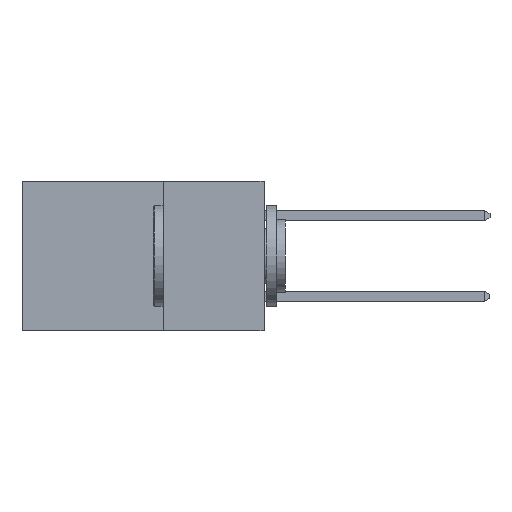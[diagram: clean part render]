
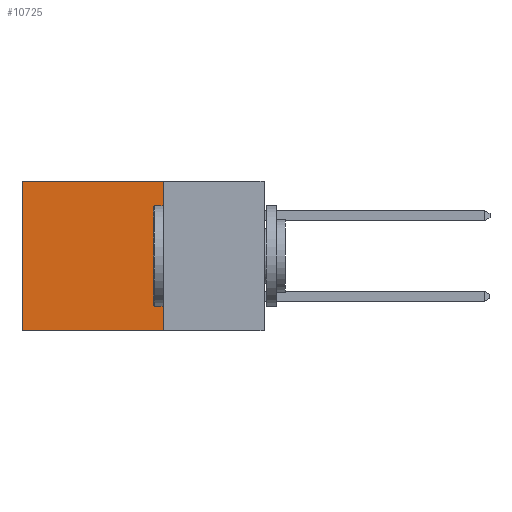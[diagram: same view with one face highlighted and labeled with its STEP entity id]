
A CAD part, left-side view. The second image highlights one B-rep face of the part: STEP entity #10725.
In plain terms, the highlighted planar face has unit normal (-1, 0, 0).
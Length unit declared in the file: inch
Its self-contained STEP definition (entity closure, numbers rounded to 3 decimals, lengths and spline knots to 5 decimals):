
#229 = DIRECTION ( 'NONE',  ( 0., 0., -1. ) ) ;
#1566 = CARTESIAN_POINT ( 'NONE',  ( 0.298, 0.25, 0. ) ) ;
#3342 = VECTOR ( 'NONE', #15782, 39.37008 ) ;
#3769 = LINE ( 'NONE', #6173, #3342 ) ;
#4072 = DIRECTION ( 'NONE',  ( 0., 1., 0. ) ) ;
#4137 = EDGE_CURVE ( 'NONE', #8385, #11185, #16039, .T. ) ;
#5126 = CARTESIAN_POINT ( 'NONE',  ( 0.298, 0.25, 0. ) ) ;
#6173 = CARTESIAN_POINT ( 'NONE',  ( 0.298, 0.6, 0. ) ) ;
#6237 = FACE_OUTER_BOUND ( 'NONE', #8114, .T. ) ;
#6563 = DIRECTION ( 'NONE',  ( 0., 0., -1. ) ) ;
#7014 = CARTESIAN_POINT ( 'NONE',  ( 0.298, 0.6, -0.37 ) ) ;
#7054 = LINE ( 'NONE', #11032, #10706 ) ;
#7848 = ORIENTED_EDGE ( 'NONE', *, *, #14014, .T. ) ;
#8114 = EDGE_LOOP ( 'NONE', ( #7848, #8485, #8613, #9883 ) ) ;
#8181 = CARTESIAN_POINT ( 'NONE',  ( 0.298, 0.25, -0.37 ) ) ;
#8225 = VECTOR ( 'NONE', #13657, 39.37008 ) ;
#8385 = VERTEX_POINT ( 'NONE', #1566 ) ;
#8485 = ORIENTED_EDGE ( 'NONE', *, *, #12906, .F. ) ;
#8613 = ORIENTED_EDGE ( 'NONE', *, *, #4137, .F. ) ;
#8800 = VECTOR ( 'NONE', #229, 39.37008 ) ;
#9276 = PLANE ( 'NONE',  #17510 ) ;
#9883 = ORIENTED_EDGE ( 'NONE', *, *, #11575, .T. ) ;
#10127 = CARTESIAN_POINT ( 'NONE',  ( 0.298, 0.25, -0.37 ) ) ;
#10706 = VECTOR ( 'NONE', #4072, 39.37008 ) ;
#10725 = ADVANCED_FACE ( 'NONE', ( #6237 ), #9276, .F. ) ;
#10964 = VERTEX_POINT ( 'NONE', #7014 ) ;
#11032 = CARTESIAN_POINT ( 'NONE',  ( 0.298, 0.25, 0. ) ) ;
#11185 = VERTEX_POINT ( 'NONE', #10127 ) ;
#11575 = EDGE_CURVE ( 'NONE', #8385, #17642, #7054, .T. ) ;
#11868 = LINE ( 'NONE', #8181, #8225 ) ;
#12499 = CARTESIAN_POINT ( 'NONE',  ( 0.298, 0.25, 0. ) ) ;
#12906 = EDGE_CURVE ( 'NONE', #11185, #10964, #11868, .T. ) ;
#13657 = DIRECTION ( 'NONE',  ( 0., 1., 0. ) ) ;
#14014 = EDGE_CURVE ( 'NONE', #17642, #10964, #3769, .T. ) ;
#14725 = DIRECTION ( 'NONE',  ( 1., 0., 0. ) ) ;
#15342 = CARTESIAN_POINT ( 'NONE',  ( 0.298, 0.6, 0. ) ) ;
#15782 = DIRECTION ( 'NONE',  ( 0., 0., -1. ) ) ;
#16039 = LINE ( 'NONE', #12499, #8800 ) ;
#17510 = AXIS2_PLACEMENT_3D ( 'NONE', #5126, #14725, #6563 ) ;
#17642 = VERTEX_POINT ( 'NONE', #15342 ) ;
